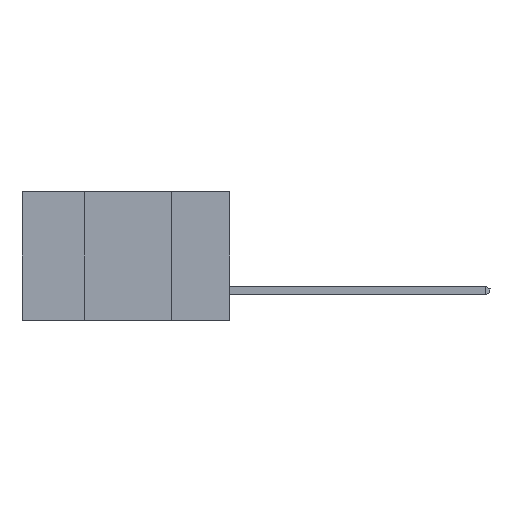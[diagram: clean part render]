
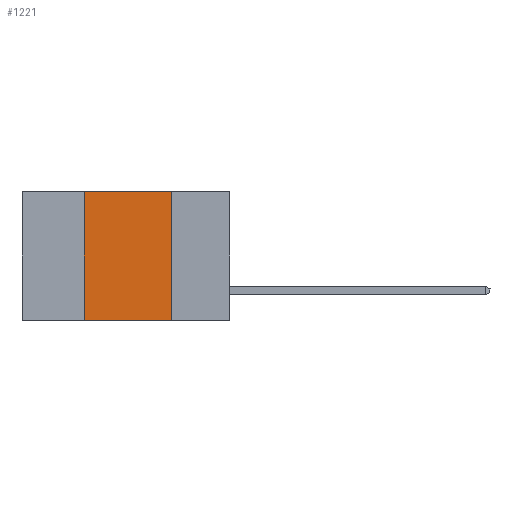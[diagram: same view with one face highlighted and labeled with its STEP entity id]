
A CAD part, left-side view. The second image highlights one B-rep face of the part: STEP entity #1221.
In plain terms, the highlighted planar face has unit normal (-1, 0, 0).
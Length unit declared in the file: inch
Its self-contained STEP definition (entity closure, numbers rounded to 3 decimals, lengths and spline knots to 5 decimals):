
#90 = ORIENTED_EDGE ( 'NONE', *, *, #7719, .T. ) ;
#603 = VECTOR ( 'NONE', #10601, 39.37008 ) ;
#709 = ORIENTED_EDGE ( 'NONE', *, *, #7011, .F. ) ;
#990 = LINE ( 'NONE', #9059, #9490 ) ;
#1221 = ADVANCED_FACE ( 'NONE', ( #13243 ), #9518, .F. ) ;
#1272 = EDGE_CURVE ( 'NONE', #9398, #7835, #11922, .T. ) ;
#1780 = ORIENTED_EDGE ( 'NONE', *, *, #11285, .F. ) ;
#2055 = VECTOR ( 'NONE', #2946, 39.37008 ) ;
#2480 = LINE ( 'NONE', #4794, #603 ) ;
#2661 = CARTESIAN_POINT ( 'NONE',  ( 0., 0.42, -0.37 ) ) ;
#2946 = DIRECTION ( 'NONE',  ( 0., 0., -1. ) ) ;
#3381 = DIRECTION ( 'NONE',  ( 0., 0., 1. ) ) ;
#4209 = LINE ( 'NONE', #5348, #2055 ) ;
#4475 = CARTESIAN_POINT ( 'NONE',  ( 0., 0.42, 0. ) ) ;
#4748 = VECTOR ( 'NONE', #10945, 39.37008 ) ;
#4794 = CARTESIAN_POINT ( 'NONE',  ( 0., 0.6, -0.37 ) ) ;
#5063 = DIRECTION ( 'NONE',  ( 0., 0., -1. ) ) ;
#5124 = EDGE_LOOP ( 'NONE', ( #709, #8227, #1780, #90 ) ) ;
#5235 = VERTEX_POINT ( 'NONE', #12564 ) ;
#5348 = CARTESIAN_POINT ( 'NONE',  ( 0., 0.17, -0.37 ) ) ;
#5475 = AXIS2_PLACEMENT_3D ( 'NONE', #12946, #9592, #5063 ) ;
#7011 = EDGE_CURVE ( 'NONE', #7835, #5235, #4209, .T. ) ;
#7719 = EDGE_CURVE ( 'NONE', #8115, #5235, #2480, .T. ) ;
#7835 = VERTEX_POINT ( 'NONE', #12224 ) ;
#8115 = VERTEX_POINT ( 'NONE', #2661 ) ;
#8227 = ORIENTED_EDGE ( 'NONE', *, *, #1272, .F. ) ;
#9059 = CARTESIAN_POINT ( 'NONE',  ( 0., 0.42, -0.37 ) ) ;
#9398 = VERTEX_POINT ( 'NONE', #4475 ) ;
#9490 = VECTOR ( 'NONE', #3381, 39.37008 ) ;
#9518 = PLANE ( 'NONE',  #5475 ) ;
#9592 = DIRECTION ( 'NONE',  ( 1., 0., 0. ) ) ;
#10601 = DIRECTION ( 'NONE',  ( 0., -1., 0. ) ) ;
#10945 = DIRECTION ( 'NONE',  ( 0., -1., 0. ) ) ;
#11285 = EDGE_CURVE ( 'NONE', #8115, #9398, #990, .T. ) ;
#11922 = LINE ( 'NONE', #13095, #4748 ) ;
#12224 = CARTESIAN_POINT ( 'NONE',  ( 0., 0.17, 0. ) ) ;
#12564 = CARTESIAN_POINT ( 'NONE',  ( 0., 0.17, -0.37 ) ) ;
#12946 = CARTESIAN_POINT ( 'NONE',  ( 0., 0.6, 0. ) ) ;
#13095 = CARTESIAN_POINT ( 'NONE',  ( 0., 0.6, 0. ) ) ;
#13243 = FACE_OUTER_BOUND ( 'NONE', #5124, .T. ) ;
